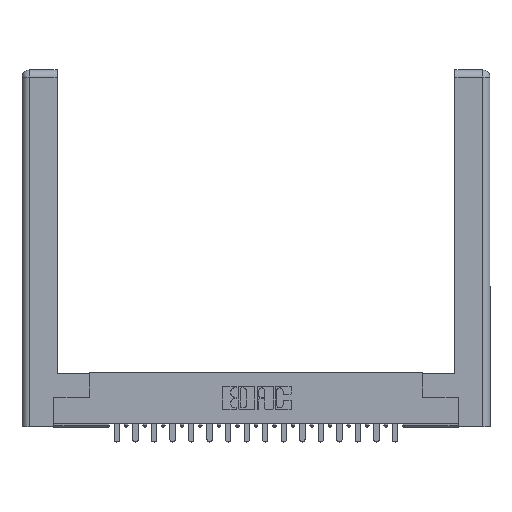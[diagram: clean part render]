
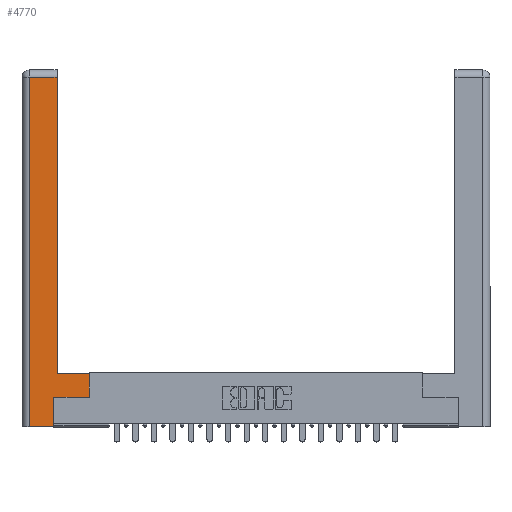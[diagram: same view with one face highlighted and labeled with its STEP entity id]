
A CAD part, top view. The second image highlights one B-rep face of the part: STEP entity #4770.
In plain terms, the highlighted planar face has unit normal (0, 0, 1).
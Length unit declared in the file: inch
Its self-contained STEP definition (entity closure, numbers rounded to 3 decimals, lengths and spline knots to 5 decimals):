
#66 = LINE ( 'NONE', #5282, #2532 ) ;
#163 = EDGE_LOOP ( 'NONE', ( #21975, #17568, #21629, #11081, #4454, #4847, #22581, #15195 ) ) ;
#586 = VECTOR ( 'NONE', #9150, 39.37008 ) ;
#667 = CARTESIAN_POINT ( 'NONE',  ( 0.0615, 2.94, 0. ) ) ;
#1130 = CARTESIAN_POINT ( 'NONE',  ( 0.0615, 0., 0. ) ) ;
#1294 = DIRECTION ( 'NONE',  ( -1., 0., 0. ) ) ;
#1892 = LINE ( 'NONE', #3532, #9079 ) ;
#2067 = EDGE_CURVE ( 'NONE', #10615, #15593, #4809, .T. ) ;
#2532 = VECTOR ( 'NONE', #13976, 39.37008 ) ;
#2722 = CARTESIAN_POINT ( 'NONE',  ( 0., 0., 0. ) ) ;
#2902 = EDGE_CURVE ( 'NONE', #15324, #13515, #66, .T. ) ;
#3222 = EDGE_CURVE ( 'NONE', #19865, #18145, #6973, .T. ) ;
#3532 = CARTESIAN_POINT ( 'NONE',  ( 0.565, 0.45, 0. ) ) ;
#4076 = LINE ( 'NONE', #18172, #13538 ) ;
#4454 = ORIENTED_EDGE ( 'NONE', *, *, #2902, .T. ) ;
#4494 = CARTESIAN_POINT ( 'NONE',  ( 0.565, 0.245, 0. ) ) ;
#4639 = VERTEX_POINT ( 'NONE', #5160 ) ;
#4770 = ADVANCED_FACE ( 'NONE', ( #5502 ), #10084, .F. ) ;
#4809 = LINE ( 'NONE', #21701, #13691 ) ;
#4847 = ORIENTED_EDGE ( 'NONE', *, *, #22777, .T. ) ;
#5160 = CARTESIAN_POINT ( 'NONE',  ( 0.295, 2.94, 0. ) ) ;
#5178 = CARTESIAN_POINT ( 'NONE',  ( 0.295, 0.45, 0. ) ) ;
#5282 = CARTESIAN_POINT ( 'NONE',  ( 0.265, 0.245, 0. ) ) ;
#5502 = FACE_OUTER_BOUND ( 'NONE', #163, .T. ) ;
#5565 = CARTESIAN_POINT ( 'NONE',  ( 0.265, 0.245, 0. ) ) ;
#5596 = CARTESIAN_POINT ( 'NONE',  ( 0.0615, 0., 0. ) ) ;
#6453 = DIRECTION ( 'NONE',  ( 0., 0., -1. ) ) ;
#6643 = CARTESIAN_POINT ( 'NONE',  ( 0.295, 3., 0. ) ) ;
#6973 = LINE ( 'NONE', #5596, #586 ) ;
#7144 = DIRECTION ( 'NONE',  ( 0., 1., 0. ) ) ;
#9079 = VECTOR ( 'NONE', #7144, 39.37008 ) ;
#9150 = DIRECTION ( 'NONE',  ( 0., -1., 0. ) ) ;
#10073 = LINE ( 'NONE', #667, #18691 ) ;
#10084 = PLANE ( 'NONE',  #18921 ) ;
#10190 = CARTESIAN_POINT ( 'NONE',  ( 0.565, 0.45, 0. ) ) ;
#10615 = VERTEX_POINT ( 'NONE', #10190 ) ;
#11081 = ORIENTED_EDGE ( 'NONE', *, *, #21838, .T. ) ;
#13483 = VECTOR ( 'NONE', #13784, 39.37008 ) ;
#13515 = VERTEX_POINT ( 'NONE', #5565 ) ;
#13538 = VECTOR ( 'NONE', #19927, 39.37008 ) ;
#13691 = VECTOR ( 'NONE', #18317, 39.37008 ) ;
#13784 = DIRECTION ( 'NONE',  ( 0., 1., 0. ) ) ;
#13976 = DIRECTION ( 'NONE',  ( 0., 1., 0. ) ) ;
#15195 = ORIENTED_EDGE ( 'NONE', *, *, #2067, .T. ) ;
#15203 = VERTEX_POINT ( 'NONE', #4494 ) ;
#15231 = DIRECTION ( 'NONE',  ( -1., 0., 0. ) ) ;
#15324 = VERTEX_POINT ( 'NONE', #15530 ) ;
#15530 = CARTESIAN_POINT ( 'NONE',  ( 0.265, 0., 0. ) ) ;
#15593 = VERTEX_POINT ( 'NONE', #5178 ) ;
#15846 = CARTESIAN_POINT ( 'NONE',  ( 0.0615, 2.94, 0. ) ) ;
#16155 = EDGE_CURVE ( 'NONE', #4639, #19865, #10073, .T. ) ;
#16897 = VECTOR ( 'NONE', #17781, 39.37008 ) ;
#17568 = ORIENTED_EDGE ( 'NONE', *, *, #16155, .T. ) ;
#17781 = DIRECTION ( 'NONE',  ( 1., 0., 0. ) ) ;
#18145 = VERTEX_POINT ( 'NONE', #1130 ) ;
#18155 = LINE ( 'NONE', #6643, #13483 ) ;
#18172 = CARTESIAN_POINT ( 'NONE',  ( 0.565, 0.245, 0. ) ) ;
#18317 = DIRECTION ( 'NONE',  ( -1., 0., 0. ) ) ;
#18691 = VECTOR ( 'NONE', #1294, 39.37008 ) ;
#18921 = AXIS2_PLACEMENT_3D ( 'NONE', #2722, #6453, #15231 ) ;
#19128 = EDGE_CURVE ( 'NONE', #15203, #10615, #1892, .T. ) ;
#19151 = LINE ( 'NONE', #21613, #16897 ) ;
#19865 = VERTEX_POINT ( 'NONE', #15846 ) ;
#19927 = DIRECTION ( 'NONE',  ( 1., 0., 0. ) ) ;
#20804 = EDGE_CURVE ( 'NONE', #15593, #4639, #18155, .T. ) ;
#21613 = CARTESIAN_POINT ( 'NONE',  ( 0.265, 0., 0. ) ) ;
#21629 = ORIENTED_EDGE ( 'NONE', *, *, #3222, .T. ) ;
#21701 = CARTESIAN_POINT ( 'NONE',  ( 0.295, 0.45, 0. ) ) ;
#21838 = EDGE_CURVE ( 'NONE', #18145, #15324, #19151, .T. ) ;
#21975 = ORIENTED_EDGE ( 'NONE', *, *, #20804, .T. ) ;
#22581 = ORIENTED_EDGE ( 'NONE', *, *, #19128, .T. ) ;
#22777 = EDGE_CURVE ( 'NONE', #13515, #15203, #4076, .T. ) ;
